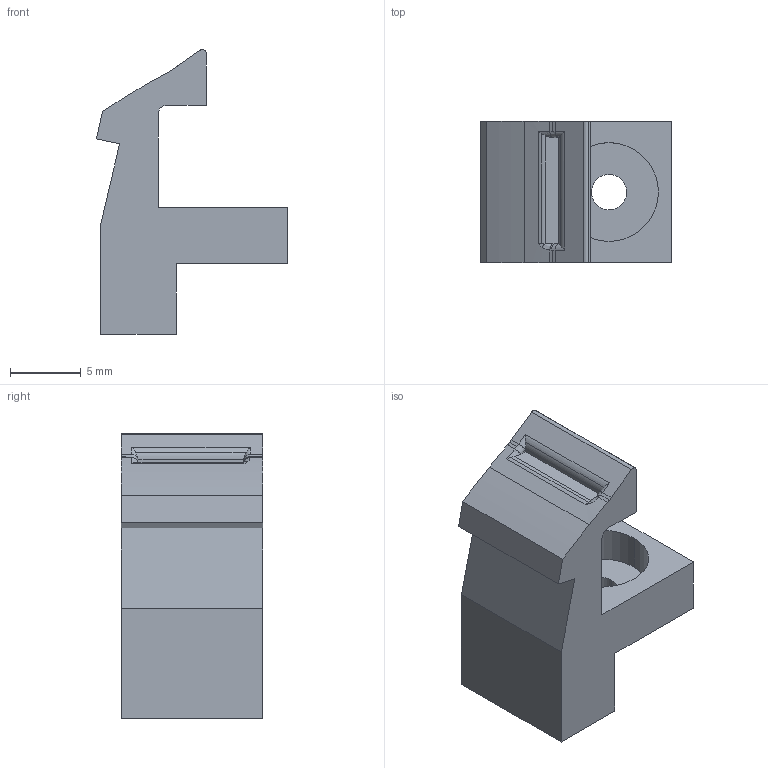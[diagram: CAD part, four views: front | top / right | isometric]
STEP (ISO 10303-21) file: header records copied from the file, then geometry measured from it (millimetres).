
FILE_DESCRIPTION(('STEP AP214'),'1');
FILE_NAME('MOD9E Feed Ramp.stp','2020-09-01T22:16:24',(' '),(' '),'Spatial InterOp 3D',' ',' ');
FILE_SCHEMA(('AUTOMOTIVE_DESIGN { 1 0 10303 214 1 1 1 1 }'));
Length unit declared in the file: metre
Products named in the file (1): Solid1
Bounding box: 13.52 x 10 x 20.16 mm (x, y, z)
Volume: 1080.2 mm3; surface area: 1013.4 mm2
Topology: 1 solids, 1 shells, 46 faces, 124 edges, 80 vertices
Faces by surface type: cylinder 20, plane 20, bspline 6
Entity records: 2614 total; most frequent: CARTESIAN_POINT 1456, ORIENTED_EDGE 246, DIRECTION 221, EDGE_CURVE 123, VERTEX_POINT 80, AXIS2_PLACEMENT_3D 75, LINE 71, VECTOR 71
